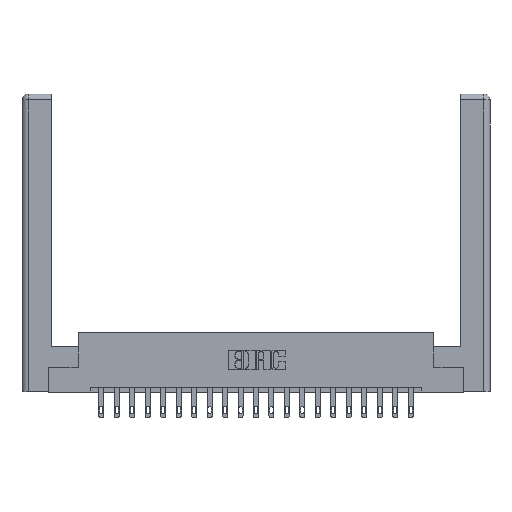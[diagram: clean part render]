
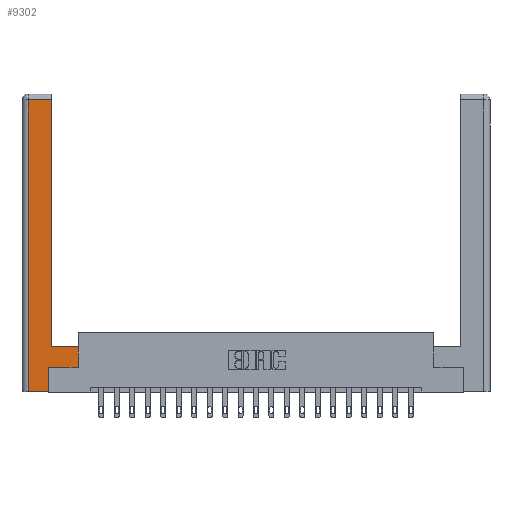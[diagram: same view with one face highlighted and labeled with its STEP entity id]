
A CAD part, top view. The second image highlights one B-rep face of the part: STEP entity #9302.
In plain terms, the highlighted planar face has unit normal (0, 0, 1).
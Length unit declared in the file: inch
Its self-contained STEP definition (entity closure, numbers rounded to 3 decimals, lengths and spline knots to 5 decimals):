
#168 = LINE ( 'NONE', #18976, #6730 ) ;
#256 = LINE ( 'NONE', #14451, #20347 ) ;
#456 = CARTESIAN_POINT ( 'NONE',  ( 0.565, 0.45, 0. ) ) ;
#539 = AXIS2_PLACEMENT_3D ( 'NONE', #8220, #20020, #1880 ) ;
#679 = DIRECTION ( 'NONE',  ( 0., 1., 0. ) ) ;
#763 = CARTESIAN_POINT ( 'NONE',  ( 0.0615, 2.94, 0. ) ) ;
#1195 = DIRECTION ( 'NONE',  ( 0., 1., 0. ) ) ;
#1518 = PLANE ( 'NONE',  #539 ) ;
#1852 = ORIENTED_EDGE ( 'NONE', *, *, #15008, .T. ) ;
#1875 = ORIENTED_EDGE ( 'NONE', *, *, #4533, .T. ) ;
#1880 = DIRECTION ( 'NONE',  ( -1., 0., 0. ) ) ;
#2294 = CARTESIAN_POINT ( 'NONE',  ( 0.265, 0.245, 0. ) ) ;
#2328 = DIRECTION ( 'NONE',  ( -1., 0., 0. ) ) ;
#2517 = DIRECTION ( 'NONE',  ( -1., 0., 0. ) ) ;
#2659 = CARTESIAN_POINT ( 'NONE',  ( 0.0615, 2.94, 0. ) ) ;
#3230 = CARTESIAN_POINT ( 'NONE',  ( 0.565, 0.245, 0. ) ) ;
#3470 = VERTEX_POINT ( 'NONE', #5350 ) ;
#4321 = CARTESIAN_POINT ( 'NONE',  ( 0.0615, 0., 0. ) ) ;
#4455 = ORIENTED_EDGE ( 'NONE', *, *, #15800, .T. ) ;
#4533 = EDGE_CURVE ( 'NONE', #16932, #5591, #9640, .T. ) ;
#4697 = VECTOR ( 'NONE', #12129, 39.37008 ) ;
#5333 = LINE ( 'NONE', #4321, #12634 ) ;
#5350 = CARTESIAN_POINT ( 'NONE',  ( 0.295, 2.94, 0. ) ) ;
#5591 = VERTEX_POINT ( 'NONE', #15224 ) ;
#6418 = VECTOR ( 'NONE', #2328, 39.37008 ) ;
#6525 = EDGE_CURVE ( 'NONE', #13367, #3470, #168, .T. ) ;
#6682 = DIRECTION ( 'NONE',  ( 1., 0., 0. ) ) ;
#6730 = VECTOR ( 'NONE', #679, 39.37008 ) ;
#7265 = ORIENTED_EDGE ( 'NONE', *, *, #6525, .T. ) ;
#7665 = EDGE_CURVE ( 'NONE', #3470, #12414, #12655, .T. ) ;
#7751 = DIRECTION ( 'NONE',  ( 0., -1., 0. ) ) ;
#7916 = EDGE_CURVE ( 'NONE', #18427, #15426, #7952, .T. ) ;
#7952 = LINE ( 'NONE', #19930, #16808 ) ;
#8217 = LINE ( 'NONE', #15977, #20461 ) ;
#8220 = CARTESIAN_POINT ( 'NONE',  ( 0., 0., 0. ) ) ;
#8384 = EDGE_CURVE ( 'NONE', #12414, #18427, #5333, .T. ) ;
#9302 = ADVANCED_FACE ( 'NONE', ( #18062 ), #1518, .F. ) ;
#9640 = LINE ( 'NONE', #456, #4697 ) ;
#10336 = ORIENTED_EDGE ( 'NONE', *, *, #7916, .T. ) ;
#12129 = DIRECTION ( 'NONE',  ( 0., 1., 0. ) ) ;
#12414 = VERTEX_POINT ( 'NONE', #2659 ) ;
#12634 = VECTOR ( 'NONE', #7751, 39.37008 ) ;
#12655 = LINE ( 'NONE', #763, #6418 ) ;
#12918 = ORIENTED_EDGE ( 'NONE', *, *, #18084, .T. ) ;
#13336 = DIRECTION ( 'NONE',  ( 1., 0., 0. ) ) ;
#13367 = VERTEX_POINT ( 'NONE', #17129 ) ;
#14451 = CARTESIAN_POINT ( 'NONE',  ( 0.265, 0.245, 0. ) ) ;
#14580 = VECTOR ( 'NONE', #13336, 39.37008 ) ;
#15008 = EDGE_CURVE ( 'NONE', #15426, #17968, #256, .T. ) ;
#15224 = CARTESIAN_POINT ( 'NONE',  ( 0.565, 0.45, 0. ) ) ;
#15426 = VERTEX_POINT ( 'NONE', #17499 ) ;
#15800 = EDGE_CURVE ( 'NONE', #17968, #16932, #18255, .T. ) ;
#15977 = CARTESIAN_POINT ( 'NONE',  ( 0.295, 0.45, 0. ) ) ;
#16325 = ORIENTED_EDGE ( 'NONE', *, *, #7665, .T. ) ;
#16479 = EDGE_LOOP ( 'NONE', ( #7265, #16325, #17318, #10336, #1852, #4455, #1875, #12918 ) ) ;
#16808 = VECTOR ( 'NONE', #6682, 39.37008 ) ;
#16932 = VERTEX_POINT ( 'NONE', #19734 ) ;
#17129 = CARTESIAN_POINT ( 'NONE',  ( 0.295, 0.45, 0. ) ) ;
#17318 = ORIENTED_EDGE ( 'NONE', *, *, #8384, .T. ) ;
#17499 = CARTESIAN_POINT ( 'NONE',  ( 0.265, 0., 0. ) ) ;
#17968 = VERTEX_POINT ( 'NONE', #2294 ) ;
#18062 = FACE_OUTER_BOUND ( 'NONE', #16479, .T. ) ;
#18084 = EDGE_CURVE ( 'NONE', #5591, #13367, #8217, .T. ) ;
#18255 = LINE ( 'NONE', #3230, #14580 ) ;
#18427 = VERTEX_POINT ( 'NONE', #20315 ) ;
#18976 = CARTESIAN_POINT ( 'NONE',  ( 0.295, 3., 0. ) ) ;
#19734 = CARTESIAN_POINT ( 'NONE',  ( 0.565, 0.245, 0. ) ) ;
#19930 = CARTESIAN_POINT ( 'NONE',  ( 0.265, 0., 0. ) ) ;
#20020 = DIRECTION ( 'NONE',  ( 0., 0., -1. ) ) ;
#20315 = CARTESIAN_POINT ( 'NONE',  ( 0.0615, 0., 0. ) ) ;
#20347 = VECTOR ( 'NONE', #1195, 39.37008 ) ;
#20461 = VECTOR ( 'NONE', #2517, 39.37008 ) ;
